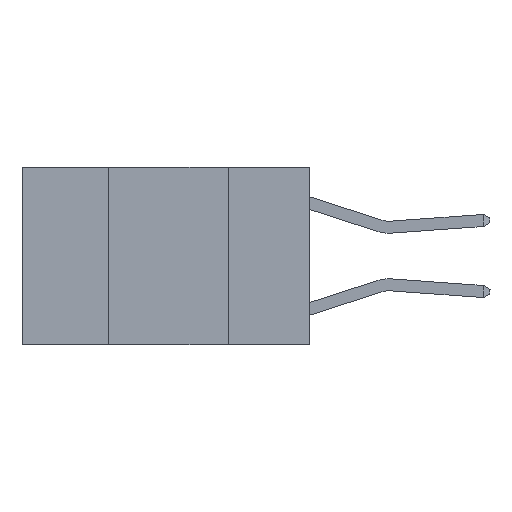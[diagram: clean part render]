
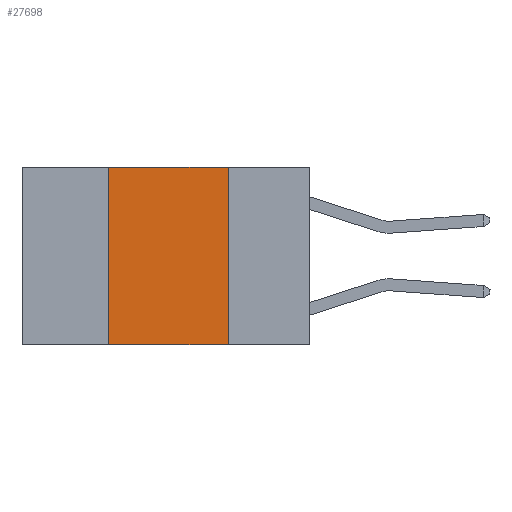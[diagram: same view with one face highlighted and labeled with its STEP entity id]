
A CAD part, left-side view. The second image highlights one B-rep face of the part: STEP entity #27698.
In plain terms, the highlighted planar face has unit normal (-1, 0, 0).
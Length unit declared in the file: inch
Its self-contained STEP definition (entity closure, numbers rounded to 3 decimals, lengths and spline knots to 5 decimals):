
#28 = LINE ( 'NONE', #21481, #6267 ) ;
#1048 = VERTEX_POINT ( 'NONE', #26769 ) ;
#1607 = CARTESIAN_POINT ( 'NONE',  ( 0., 0.42, 0. ) ) ;
#2859 = EDGE_CURVE ( 'NONE', #5569, #17860, #25583, .T. ) ;
#3002 = AXIS2_PLACEMENT_3D ( 'NONE', #27210, #23069, #12416 ) ;
#3958 = VECTOR ( 'NONE', #5388, 39.37008 ) ;
#5388 = DIRECTION ( 'NONE',  ( 0., 0., 1. ) ) ;
#5569 = VERTEX_POINT ( 'NONE', #5571 ) ;
#5571 = CARTESIAN_POINT ( 'NONE',  ( 0., 0.42, -0.37 ) ) ;
#6267 = VECTOR ( 'NONE', #12533, 39.37008 ) ;
#6400 = CARTESIAN_POINT ( 'NONE',  ( 0., 0.17, 0. ) ) ;
#7948 = ORIENTED_EDGE ( 'NONE', *, *, #2859, .T. ) ;
#10096 = DIRECTION ( 'NONE',  ( 0., -1., 0. ) ) ;
#10293 = EDGE_CURVE ( 'NONE', #5569, #17854, #15313, .T. ) ;
#11078 = CARTESIAN_POINT ( 'NONE',  ( 0., 0.42, 0. ) ) ;
#11089 = EDGE_CURVE ( 'NONE', #17854, #1048, #28, .T. ) ;
#12416 = DIRECTION ( 'NONE',  ( 0., 0., -1. ) ) ;
#12533 = DIRECTION ( 'NONE',  ( 0., -1., 0. ) ) ;
#14907 = DIRECTION ( 'NONE',  ( 0., 0., -1. ) ) ;
#14965 = CARTESIAN_POINT ( 'NONE',  ( 0., 0.17, -0.37 ) ) ;
#15313 = LINE ( 'NONE', #11078, #3958 ) ;
#16869 = CARTESIAN_POINT ( 'NONE',  ( 0., 0.6, -0.37 ) ) ;
#17205 = VECTOR ( 'NONE', #10096, 39.37008 ) ;
#17854 = VERTEX_POINT ( 'NONE', #1607 ) ;
#17860 = VERTEX_POINT ( 'NONE', #14965 ) ;
#21481 = CARTESIAN_POINT ( 'NONE',  ( 0., 0.6, 0. ) ) ;
#23069 = DIRECTION ( 'NONE',  ( 1., 0., 0. ) ) ;
#24688 = ORIENTED_EDGE ( 'NONE', *, *, #24738, .F. ) ;
#24738 = EDGE_CURVE ( 'NONE', #1048, #17860, #25602, .T. ) ;
#25358 = PLANE ( 'NONE',  #3002 ) ;
#25421 = ORIENTED_EDGE ( 'NONE', *, *, #11089, .F. ) ;
#25583 = LINE ( 'NONE', #16869, #17205 ) ;
#25602 = LINE ( 'NONE', #6400, #27408 ) ;
#26769 = CARTESIAN_POINT ( 'NONE',  ( 0., 0.17, 0. ) ) ;
#27210 = CARTESIAN_POINT ( 'NONE',  ( 0., 0.6, 0. ) ) ;
#27245 = ORIENTED_EDGE ( 'NONE', *, *, #10293, .F. ) ;
#27325 = EDGE_LOOP ( 'NONE', ( #24688, #25421, #27245, #7948 ) ) ;
#27349 = FACE_OUTER_BOUND ( 'NONE', #27325, .T. ) ;
#27408 = VECTOR ( 'NONE', #14907, 39.37008 ) ;
#27698 = ADVANCED_FACE ( 'NONE', ( #27349 ), #25358, .F. ) ;
